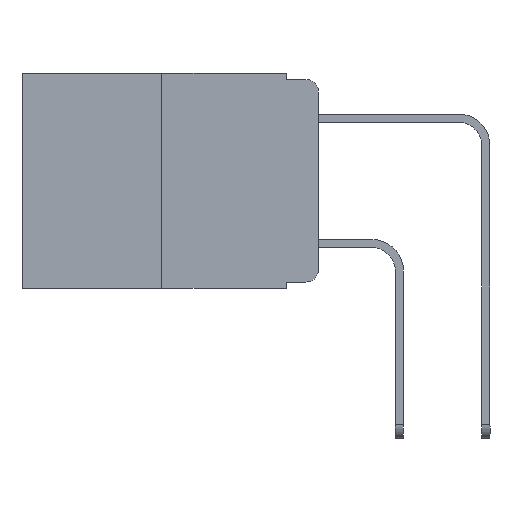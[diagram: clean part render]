
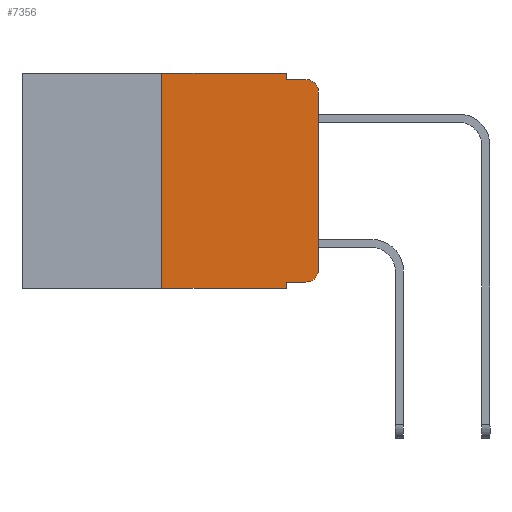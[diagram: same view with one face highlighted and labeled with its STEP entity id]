
A CAD part, left-side view. The second image highlights one B-rep face of the part: STEP entity #7356.
In plain terms, the highlighted planar face has unit normal (-1, 0, 0).
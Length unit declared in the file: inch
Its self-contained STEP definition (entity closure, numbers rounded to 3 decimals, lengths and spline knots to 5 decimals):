
#104 = FACE_OUTER_BOUND ( 'NONE', #1169, .T. ) ;
#256 = VECTOR ( 'NONE', #6364, 39.37008 ) ;
#342 = ORIENTED_EDGE ( 'NONE', *, *, #9216, .F. ) ;
#398 = LINE ( 'NONE', #7886, #9293 ) ;
#751 = CARTESIAN_POINT ( 'NONE',  ( 0., 0.02, -0.313 ) ) ;
#829 = DIRECTION ( 'NONE',  ( -1., 0., 0. ) ) ;
#1169 = EDGE_LOOP ( 'NONE', ( #13595, #9886, #17222, #4475, #9094, #12833, #5488, #342, #1812, #3271 ) ) ;
#1668 = CARTESIAN_POINT ( 'NONE',  ( 0., 0.473, 0. ) ) ;
#1812 = ORIENTED_EDGE ( 'NONE', *, *, #12608, .T. ) ;
#1963 = DIRECTION ( 'NONE',  ( 0., 0., 1. ) ) ;
#2109 = CARTESIAN_POINT ( 'NONE',  ( 0., 0.473, 0. ) ) ;
#2214 = DIRECTION ( 'NONE',  ( 0., 0., -1. ) ) ;
#2381 = CARTESIAN_POINT ( 'NONE',  ( 0., 0.02, -0.03 ) ) ;
#2669 = VERTEX_POINT ( 'NONE', #16656 ) ;
#3064 = DIRECTION ( 'NONE',  ( 0., -1., 0. ) ) ;
#3107 = PLANE ( 'NONE',  #14579 ) ;
#3184 = VERTEX_POINT ( 'NONE', #12927 ) ;
#3271 = ORIENTED_EDGE ( 'NONE', *, *, #16152, .T. ) ;
#3460 = VECTOR ( 'NONE', #1963, 39.37008 ) ;
#3590 = LINE ( 'NONE', #16069, #4948 ) ;
#3866 = CARTESIAN_POINT ( 'NONE',  ( 0., 0.051, -0.333 ) ) ;
#4362 = LINE ( 'NONE', #15729, #15464 ) ;
#4475 = ORIENTED_EDGE ( 'NONE', *, *, #11966, .F. ) ;
#4620 = LINE ( 'NONE', #9125, #3460 ) ;
#4760 = VECTOR ( 'NONE', #9345, 39.37008 ) ;
#4948 = VECTOR ( 'NONE', #2214, 39.37008 ) ;
#5488 = ORIENTED_EDGE ( 'NONE', *, *, #10525, .T. ) ;
#5683 = DIRECTION ( 'NONE',  ( 1., 0., 0. ) ) ;
#5891 = VERTEX_POINT ( 'NONE', #6611 ) ;
#6236 = LINE ( 'NONE', #2109, #4760 ) ;
#6364 = DIRECTION ( 'NONE',  ( 0., 0., -1. ) ) ;
#6414 = DIRECTION ( 'NONE',  ( 0., 0., 1. ) ) ;
#6611 = CARTESIAN_POINT ( 'NONE',  ( 0., 0.051, -0.01 ) ) ;
#6977 = VECTOR ( 'NONE', #3064, 39.37008 ) ;
#7356 = ADVANCED_FACE ( 'NONE', ( #104 ), #3107, .F. ) ;
#7886 = CARTESIAN_POINT ( 'NONE',  ( 0., 0., 0. ) ) ;
#7893 = CIRCLE ( 'NONE', #17849, 0.02 ) ;
#7989 = DIRECTION ( 'NONE',  ( 0., 0., -1. ) ) ;
#8104 = DIRECTION ( 'NONE',  ( 0., -1., 0. ) ) ;
#8359 = CARTESIAN_POINT ( 'NONE',  ( 0., 0., -0.313 ) ) ;
#8400 = LINE ( 'NONE', #9854, #6977 ) ;
#8495 = DIRECTION ( 'NONE',  ( 0., -1., 0. ) ) ;
#9094 = ORIENTED_EDGE ( 'NONE', *, *, #17495, .F. ) ;
#9125 = CARTESIAN_POINT ( 'NONE',  ( 0., 0.25, 0. ) ) ;
#9216 = EDGE_CURVE ( 'NONE', #10928, #13916, #3590, .T. ) ;
#9293 = VECTOR ( 'NONE', #6414, 39.37008 ) ;
#9338 = VECTOR ( 'NONE', #8104, 39.37008 ) ;
#9345 = DIRECTION ( 'NONE',  ( 0., -1., 0. ) ) ;
#9484 = VERTEX_POINT ( 'NONE', #8359 ) ;
#9779 = VERTEX_POINT ( 'NONE', #17598 ) ;
#9854 = CARTESIAN_POINT ( 'NONE',  ( 0., 0.473, -0.343 ) ) ;
#9886 = ORIENTED_EDGE ( 'NONE', *, *, #12973, .T. ) ;
#10313 = CARTESIAN_POINT ( 'NONE',  ( 0., 0.051, 0. ) ) ;
#10332 = AXIS2_PLACEMENT_3D ( 'NONE', #751, #10733, #12109 ) ;
#10525 = EDGE_CURVE ( 'NONE', #14198, #13916, #8400, .T. ) ;
#10571 = EDGE_CURVE ( 'NONE', #14198, #3184, #4620, .T. ) ;
#10617 = CIRCLE ( 'NONE', #10332, 0.02 ) ;
#10733 = DIRECTION ( 'NONE',  ( -1., 0., 0. ) ) ;
#10928 = VERTEX_POINT ( 'NONE', #15614 ) ;
#10948 = CARTESIAN_POINT ( 'NONE',  ( 0., 0.25, -0.343 ) ) ;
#11051 = EDGE_CURVE ( 'NONE', #9484, #11587, #398, .T. ) ;
#11587 = VERTEX_POINT ( 'NONE', #15275 ) ;
#11699 = CARTESIAN_POINT ( 'NONE',  ( 0., 0.051, -0.343 ) ) ;
#11766 = EDGE_CURVE ( 'NONE', #5891, #12845, #4362, .T. ) ;
#11872 = LINE ( 'NONE', #10313, #256 ) ;
#11917 = CARTESIAN_POINT ( 'NONE',  ( 0., 0.02, -0.01 ) ) ;
#11966 = EDGE_CURVE ( 'NONE', #2669, #5891, #11872, .T. ) ;
#12109 = DIRECTION ( 'NONE',  ( 0., 0., -1. ) ) ;
#12117 = LINE ( 'NONE', #3866, #9338 ) ;
#12608 = EDGE_CURVE ( 'NONE', #10928, #9779, #12117, .T. ) ;
#12833 = ORIENTED_EDGE ( 'NONE', *, *, #10571, .F. ) ;
#12845 = VERTEX_POINT ( 'NONE', #11917 ) ;
#12927 = CARTESIAN_POINT ( 'NONE',  ( 0., 0.25, 0. ) ) ;
#12973 = EDGE_CURVE ( 'NONE', #11587, #12845, #7893, .T. ) ;
#13595 = ORIENTED_EDGE ( 'NONE', *, *, #11051, .T. ) ;
#13916 = VERTEX_POINT ( 'NONE', #11699 ) ;
#14198 = VERTEX_POINT ( 'NONE', #10948 ) ;
#14389 = DIRECTION ( 'NONE',  ( 0., 0., -1. ) ) ;
#14579 = AXIS2_PLACEMENT_3D ( 'NONE', #1668, #5683, #14389 ) ;
#15275 = CARTESIAN_POINT ( 'NONE',  ( 0., 0., -0.03 ) ) ;
#15464 = VECTOR ( 'NONE', #8495, 39.37008 ) ;
#15614 = CARTESIAN_POINT ( 'NONE',  ( 0., 0.051, -0.333 ) ) ;
#15729 = CARTESIAN_POINT ( 'NONE',  ( 0., 0.051, -0.01 ) ) ;
#16069 = CARTESIAN_POINT ( 'NONE',  ( 0., 0.051, 0. ) ) ;
#16152 = EDGE_CURVE ( 'NONE', #9779, #9484, #10617, .T. ) ;
#16656 = CARTESIAN_POINT ( 'NONE',  ( 0., 0.051, 0. ) ) ;
#17222 = ORIENTED_EDGE ( 'NONE', *, *, #11766, .F. ) ;
#17495 = EDGE_CURVE ( 'NONE', #3184, #2669, #6236, .T. ) ;
#17598 = CARTESIAN_POINT ( 'NONE',  ( 0., 0.02, -0.333 ) ) ;
#17849 = AXIS2_PLACEMENT_3D ( 'NONE', #2381, #829, #7989 ) ;
